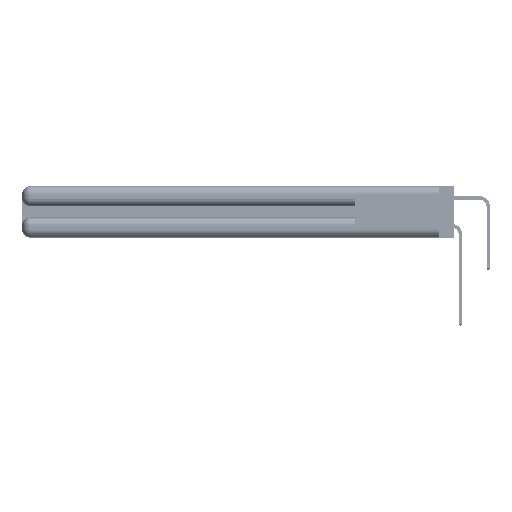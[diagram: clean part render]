
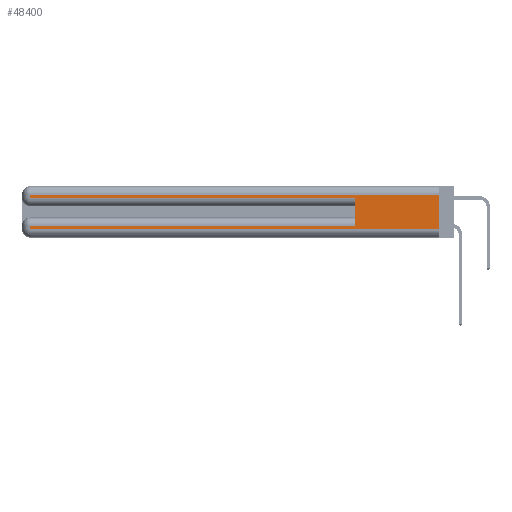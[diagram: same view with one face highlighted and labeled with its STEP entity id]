
A CAD part, left-side view. The second image highlights one B-rep face of the part: STEP entity #48400.
In plain terms, the highlighted planar face has unit normal (-1, 0, 0).
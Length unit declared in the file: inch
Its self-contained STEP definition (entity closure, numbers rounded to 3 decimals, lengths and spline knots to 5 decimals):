
#539 = CARTESIAN_POINT ( 'NONE',  ( 0., 0.6, 0.145 ) ) ;
#1614 = CARTESIAN_POINT ( 'NONE',  ( 0., 2.94, 0.37 ) ) ;
#1805 = PLANE ( 'NONE',  #5531 ) ;
#2324 = VERTEX_POINT ( 'NONE', #39753 ) ;
#4279 = LINE ( 'NONE', #1614, #22704 ) ;
#5531 = AXIS2_PLACEMENT_3D ( 'NONE', #29163, #5758, #33331 ) ;
#5758 = DIRECTION ( 'NONE',  ( 1., 0., 0. ) ) ;
#5943 = ORIENTED_EDGE ( 'NONE', *, *, #27753, .T. ) ;
#7822 = DIRECTION ( 'NONE',  ( 0., 1., 0. ) ) ;
#8788 = VECTOR ( 'NONE', #40009, 39.37008 ) ;
#8807 = ORIENTED_EDGE ( 'NONE', *, *, #19187, .T. ) ;
#9660 = VERTEX_POINT ( 'NONE', #9902 ) ;
#9902 = CARTESIAN_POINT ( 'NONE',  ( 0., 2.94, 0.085 ) ) ;
#11145 = ORIENTED_EDGE ( 'NONE', *, *, #29571, .T. ) ;
#11862 = CARTESIAN_POINT ( 'NONE',  ( 0., 0., 0.37 ) ) ;
#11868 = EDGE_LOOP ( 'NONE', ( #40182, #50161, #11145, #15678, #45704, #8807, #41490, #5943 ) ) ;
#13116 = CARTESIAN_POINT ( 'NONE',  ( 0., 0., 0.31 ) ) ;
#13442 = DIRECTION ( 'NONE',  ( 0., 0., -1. ) ) ;
#13505 = VECTOR ( 'NONE', #48695, 39.37008 ) ;
#15678 = ORIENTED_EDGE ( 'NONE', *, *, #31167, .T. ) ;
#15802 = DIRECTION ( 'NONE',  ( 0., 0., -1. ) ) ;
#16805 = EDGE_CURVE ( 'NONE', #19418, #44868, #21761, .T. ) ;
#18048 = DIRECTION ( 'NONE',  ( 0., 0., -1. ) ) ;
#18284 = VECTOR ( 'NONE', #47697, 39.37008 ) ;
#19187 = EDGE_CURVE ( 'NONE', #45599, #9660, #27074, .T. ) ;
#19418 = VERTEX_POINT ( 'NONE', #13116 ) ;
#19483 = EDGE_CURVE ( 'NONE', #9660, #43062, #4279, .T. ) ;
#19498 = LINE ( 'NONE', #31707, #18284 ) ;
#19635 = CARTESIAN_POINT ( 'NONE',  ( 0., 0., 0.085 ) ) ;
#21761 = LINE ( 'NONE', #11862, #22998 ) ;
#22704 = VECTOR ( 'NONE', #13442, 39.37008 ) ;
#22998 = VECTOR ( 'NONE', #15802, 39.37008 ) ;
#24536 = VECTOR ( 'NONE', #18048, 39.37008 ) ;
#25079 = CARTESIAN_POINT ( 'NONE',  ( 0., 0., 0.06 ) ) ;
#25863 = CARTESIAN_POINT ( 'NONE',  ( 0., 0.6, 0.285 ) ) ;
#26515 = CARTESIAN_POINT ( 'NONE',  ( 0., 0., 0.285 ) ) ;
#27074 = LINE ( 'NONE', #19635, #46822 ) ;
#27753 = EDGE_CURVE ( 'NONE', #43062, #44868, #44983, .T. ) ;
#28457 = VERTEX_POINT ( 'NONE', #42873 ) ;
#29163 = CARTESIAN_POINT ( 'NONE',  ( 0., 0., 0.37 ) ) ;
#29571 = EDGE_CURVE ( 'NONE', #2324, #28457, #45543, .T. ) ;
#29735 = LINE ( 'NONE', #539, #8788 ) ;
#30496 = DIRECTION ( 'NONE',  ( 0., -1., 0. ) ) ;
#31167 = EDGE_CURVE ( 'NONE', #28457, #50540, #41739, .T. ) ;
#31426 = FACE_OUTER_BOUND ( 'NONE', #11868, .T. ) ;
#31707 = CARTESIAN_POINT ( 'NONE',  ( 0., 0., 0.31 ) ) ;
#33331 = DIRECTION ( 'NONE',  ( 0., 0., -1. ) ) ;
#33975 = CARTESIAN_POINT ( 'NONE',  ( 0., 2.94, 0.37 ) ) ;
#34142 = EDGE_CURVE ( 'NONE', #45599, #50540, #29735, .T. ) ;
#35877 = CARTESIAN_POINT ( 'NONE',  ( 0., 2.94, 0.06 ) ) ;
#39753 = CARTESIAN_POINT ( 'NONE',  ( 0., 2.94, 0.31 ) ) ;
#40009 = DIRECTION ( 'NONE',  ( 0., 0., 1. ) ) ;
#40182 = ORIENTED_EDGE ( 'NONE', *, *, #16805, .F. ) ;
#40319 = CARTESIAN_POINT ( 'NONE',  ( 0., 0.6, 0.085 ) ) ;
#41490 = ORIENTED_EDGE ( 'NONE', *, *, #19483, .T. ) ;
#41739 = LINE ( 'NONE', #26515, #49688 ) ;
#42255 = EDGE_CURVE ( 'NONE', #19418, #2324, #19498, .T. ) ;
#42873 = CARTESIAN_POINT ( 'NONE',  ( 0., 2.94, 0.285 ) ) ;
#43062 = VERTEX_POINT ( 'NONE', #35877 ) ;
#44868 = VERTEX_POINT ( 'NONE', #47740 ) ;
#44983 = LINE ( 'NONE', #25079, #13505 ) ;
#45543 = LINE ( 'NONE', #33975, #24536 ) ;
#45599 = VERTEX_POINT ( 'NONE', #40319 ) ;
#45704 = ORIENTED_EDGE ( 'NONE', *, *, #34142, .F. ) ;
#46822 = VECTOR ( 'NONE', #7822, 39.37008 ) ;
#47697 = DIRECTION ( 'NONE',  ( 0., 1., 0. ) ) ;
#47740 = CARTESIAN_POINT ( 'NONE',  ( 0., 0., 0.06 ) ) ;
#48400 = ADVANCED_FACE ( 'NONE', ( #31426 ), #1805, .F. ) ;
#48695 = DIRECTION ( 'NONE',  ( 0., -1., 0. ) ) ;
#49688 = VECTOR ( 'NONE', #30496, 39.37008 ) ;
#50161 = ORIENTED_EDGE ( 'NONE', *, *, #42255, .T. ) ;
#50540 = VERTEX_POINT ( 'NONE', #25863 ) ;
